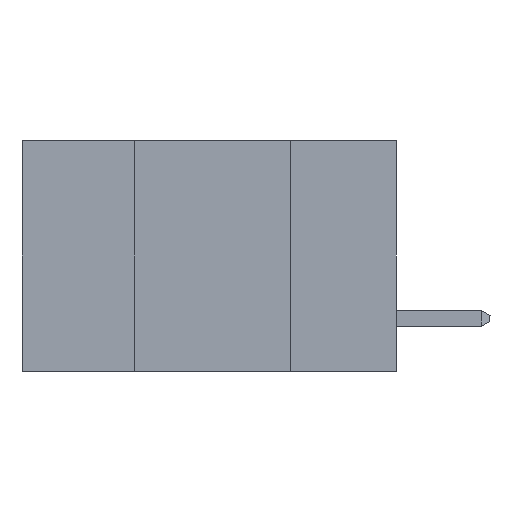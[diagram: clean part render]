
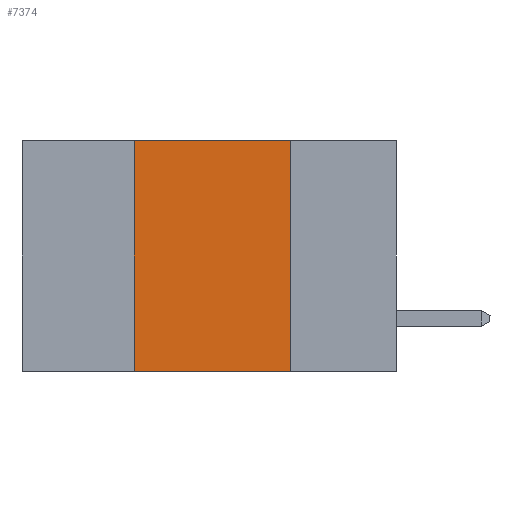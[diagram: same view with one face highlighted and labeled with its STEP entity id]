
A CAD part, left-side view. The second image highlights one B-rep face of the part: STEP entity #7374.
In plain terms, the highlighted planar face has unit normal (-1, 0, 0).
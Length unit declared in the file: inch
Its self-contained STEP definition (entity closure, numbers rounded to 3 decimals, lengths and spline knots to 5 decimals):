
#1584 = VERTEX_POINT ( 'NONE', #2955 ) ;
#1869 = EDGE_CURVE ( 'NONE', #3561, #1584, #18998, .T. ) ;
#2180 = CARTESIAN_POINT ( 'NONE',  ( 0., 0.17, -0.37 ) ) ;
#2904 = DIRECTION ( 'NONE',  ( 1., 0., 0. ) ) ;
#2955 = CARTESIAN_POINT ( 'NONE',  ( 0., 0.17, -0.37 ) ) ;
#3561 = VERTEX_POINT ( 'NONE', #20302 ) ;
#5672 = CARTESIAN_POINT ( 'NONE',  ( 0., 0.6, -0.37 ) ) ;
#6205 = CARTESIAN_POINT ( 'NONE',  ( 0., 0.42, -0.37 ) ) ;
#7267 = VECTOR ( 'NONE', #9045, 39.37008 ) ;
#7374 = ADVANCED_FACE ( 'NONE', ( #11275 ), #13128, .F. ) ;
#7383 = VERTEX_POINT ( 'NONE', #16151 ) ;
#8064 = CARTESIAN_POINT ( 'NONE',  ( 0., 0.42, -0.37 ) ) ;
#8189 = VECTOR ( 'NONE', #12826, 39.37008 ) ;
#8907 = VERTEX_POINT ( 'NONE', #8064 ) ;
#9045 = DIRECTION ( 'NONE',  ( 0., 0., -1. ) ) ;
#9161 = LINE ( 'NONE', #5672, #15709 ) ;
#11275 = FACE_OUTER_BOUND ( 'NONE', #19154, .T. ) ;
#12826 = DIRECTION ( 'NONE',  ( 0., -1., 0. ) ) ;
#13128 = PLANE ( 'NONE',  #15414 ) ;
#13646 = VECTOR ( 'NONE', #17818, 39.37008 ) ;
#13715 = DIRECTION ( 'NONE',  ( 0., -1., 0. ) ) ;
#14632 = DIRECTION ( 'NONE',  ( 0., 0., -1. ) ) ;
#15277 = ORIENTED_EDGE ( 'NONE', *, *, #16047, .F. ) ;
#15414 = AXIS2_PLACEMENT_3D ( 'NONE', #19747, #2904, #14632 ) ;
#15709 = VECTOR ( 'NONE', #13715, 39.37008 ) ;
#15925 = EDGE_CURVE ( 'NONE', #8907, #1584, #9161, .T. ) ;
#16047 = EDGE_CURVE ( 'NONE', #8907, #7383, #21219, .T. ) ;
#16119 = ORIENTED_EDGE ( 'NONE', *, *, #19418, .F. ) ;
#16151 = CARTESIAN_POINT ( 'NONE',  ( 0., 0.42, 0. ) ) ;
#17688 = LINE ( 'NONE', #19096, #8189 ) ;
#17818 = DIRECTION ( 'NONE',  ( 0., 0., 1. ) ) ;
#18985 = ORIENTED_EDGE ( 'NONE', *, *, #15925, .T. ) ;
#18998 = LINE ( 'NONE', #2180, #7267 ) ;
#19096 = CARTESIAN_POINT ( 'NONE',  ( 0., 0.6, 0. ) ) ;
#19154 = EDGE_LOOP ( 'NONE', ( #19266, #16119, #15277, #18985 ) ) ;
#19266 = ORIENTED_EDGE ( 'NONE', *, *, #1869, .F. ) ;
#19418 = EDGE_CURVE ( 'NONE', #7383, #3561, #17688, .T. ) ;
#19747 = CARTESIAN_POINT ( 'NONE',  ( 0., 0.6, 0. ) ) ;
#20302 = CARTESIAN_POINT ( 'NONE',  ( 0., 0.17, 0. ) ) ;
#21219 = LINE ( 'NONE', #6205, #13646 ) ;
